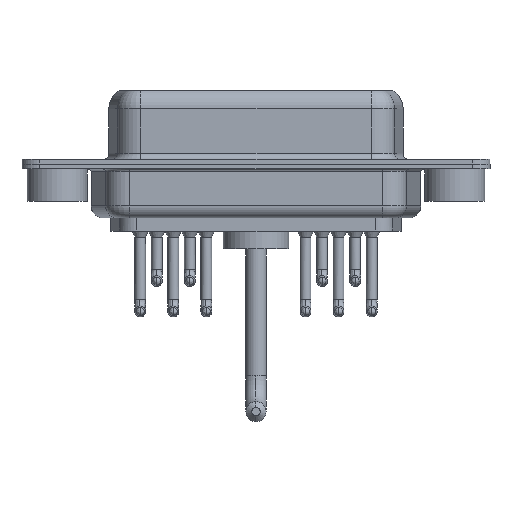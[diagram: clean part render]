
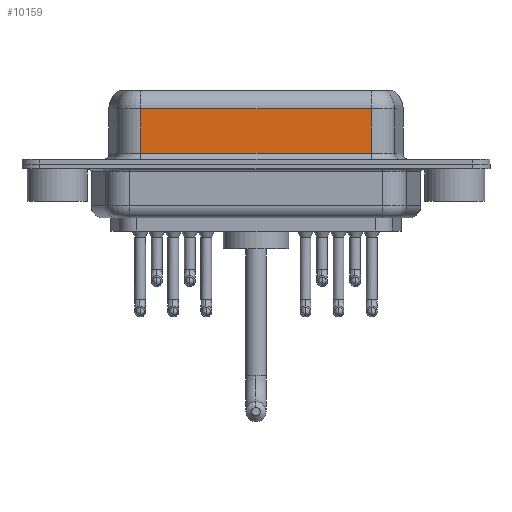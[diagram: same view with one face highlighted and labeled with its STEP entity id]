
A CAD part, front view. The second image highlights one B-rep face of the part: STEP entity #10159.
In plain terms, the highlighted planar face has unit normal (0, -1, 0).
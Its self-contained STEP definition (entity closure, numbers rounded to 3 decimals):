
#363 = DIRECTION ( 'NONE',  ( 0., 0., 1. ) ) ;
#366 = VERTEX_POINT ( 'NONE', #6987 ) ;
#385 = CARTESIAN_POINT ( 'NONE',  ( 7.013, -3.95, 4.65 ) ) ;
#1472 = ORIENTED_EDGE ( 'NONE', *, *, #7967, .T. ) ;
#1821 = LINE ( 'NONE', #2968, #6973 ) ;
#2552 = CARTESIAN_POINT ( 'NONE',  ( 26.287, -3.95, 6.4 ) ) ;
#2968 = CARTESIAN_POINT ( 'NONE',  ( 7.013, -3.95, 6.4 ) ) ;
#3473 = CARTESIAN_POINT ( 'NONE',  ( 26.287, -3.95, 6.4 ) ) ;
#3963 = EDGE_CURVE ( 'NONE', #7844, #3964, #7340, .T. ) ;
#3964 = VERTEX_POINT ( 'NONE', #385 ) ;
#4692 = DIRECTION ( 'NONE',  ( 1., 0., 0. ) ) ;
#5178 = ORIENTED_EDGE ( 'NONE', *, *, #3963, .T. ) ;
#6196 = FACE_OUTER_BOUND ( 'NONE', #13994, .T. ) ;
#6210 = LINE ( 'NONE', #16414, #15929 ) ;
#6869 = DIRECTION ( 'NONE',  ( 0., 0., -1. ) ) ;
#6973 = VECTOR ( 'NONE', #11916, 1000. ) ;
#6987 = CARTESIAN_POINT ( 'NONE',  ( 7.013, -3.95, 0.9 ) ) ;
#7340 = LINE ( 'NONE', #15745, #15514 ) ;
#7844 = VERTEX_POINT ( 'NONE', #17198 ) ;
#7967 = EDGE_CURVE ( 'NONE', #3964, #366, #1821, .T. ) ;
#9124 = PLANE ( 'NONE',  #10077 ) ;
#9221 = DIRECTION ( 'NONE',  ( 0., 1., 0. ) ) ;
#10077 = AXIS2_PLACEMENT_3D ( 'NONE', #3473, #9221, #363 ) ;
#10159 = ADVANCED_FACE ( 'NONE', ( #6196 ), #9124, .F. ) ;
#11916 = DIRECTION ( 'NONE',  ( 0., 0., -1. ) ) ;
#13994 = EDGE_LOOP ( 'NONE', ( #16529, #5178, #1472, #13997 ) ) ;
#13997 = ORIENTED_EDGE ( 'NONE', *, *, #15930, .T. ) ;
#14483 = CARTESIAN_POINT ( 'NONE',  ( 26.287, -3.95, 0.9 ) ) ;
#15514 = VECTOR ( 'NONE', #17538, 1000. ) ;
#15521 = EDGE_CURVE ( 'NONE', #7844, #16687, #16796, .T. ) ;
#15745 = CARTESIAN_POINT ( 'NONE',  ( 26.287, -3.95, 4.65 ) ) ;
#15929 = VECTOR ( 'NONE', #4692, 1000. ) ;
#15930 = EDGE_CURVE ( 'NONE', #366, #16687, #6210, .T. ) ;
#16217 = VECTOR ( 'NONE', #6869, 1000. ) ;
#16414 = CARTESIAN_POINT ( 'NONE',  ( 26.287, -3.95, 0.9 ) ) ;
#16529 = ORIENTED_EDGE ( 'NONE', *, *, #15521, .F. ) ;
#16687 = VERTEX_POINT ( 'NONE', #14483 ) ;
#16796 = LINE ( 'NONE', #2552, #16217 ) ;
#17198 = CARTESIAN_POINT ( 'NONE',  ( 26.287, -3.95, 4.65 ) ) ;
#17538 = DIRECTION ( 'NONE',  ( -1., 0., 0. ) ) ;
